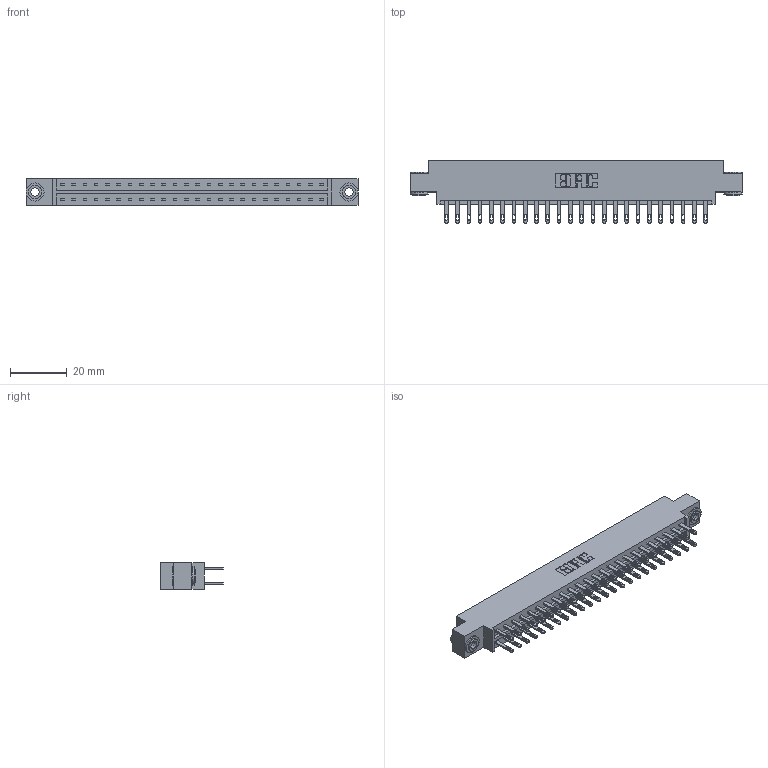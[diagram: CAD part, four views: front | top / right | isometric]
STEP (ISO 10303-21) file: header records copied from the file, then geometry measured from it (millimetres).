
FILE_DESCRIPTION (( 'STEP AP203' ), '1' );
FILE_NAME ('833-048-500-803.STEP', '2020-06-04T15:21:10', ( '' ), ( '' ), 'SwSTEP 2.0', 'SolidWorks 2020', '' );
FILE_SCHEMA (( 'CONFIG_CONTROL_DESIGN' ));
Length unit declared in the file: inch
Products named in the file (4): 345-250-002_345-250-002-102; 833 Part_Offset - .156 Dia - TH; 345-292-001_345-293-100; 833-048-500-803
Assembly tree (51 placements, depth 2):
  833-048-500-803
    833 Part_Offset - .156 Dia - TH
    345-292-001_345-293-100  x48
    345-250-002_345-250-002-102  x2
Bounding box: 116.64 x 21.85 x 9.4 mm (x, y, z)
Volume: 11677.9 mm3; surface area: 14582.7 mm2
Topology: 51 solids, 51 shells, 2460 faces, 7455 edges, 4966 vertices
Faces by surface type: plane 1524, cylinder 928, cone 8
Entity records: 18480 total; most frequent: CARTESIAN_POINT 3061, ORIENTED_EDGE 2990, DIRECTION 2681, EDGE_CURVE 1495, LINE 1339, VECTOR 1339, VERTEX_POINT 994, AXIS2_PLACEMENT_3D 671
